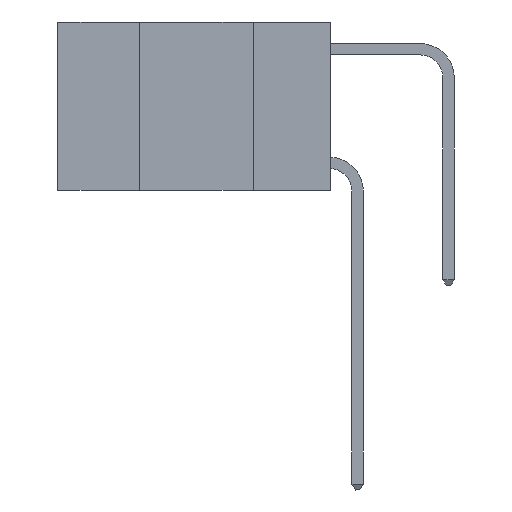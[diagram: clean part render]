
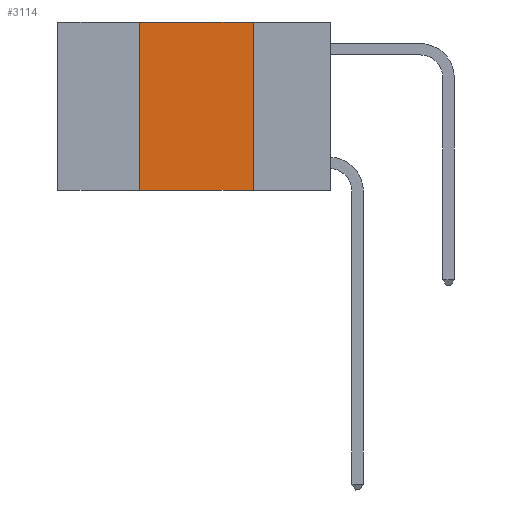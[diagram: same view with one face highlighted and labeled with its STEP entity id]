
A CAD part, left-side view. The second image highlights one B-rep face of the part: STEP entity #3114.
In plain terms, the highlighted planar face has unit normal (-1, 0, 0).
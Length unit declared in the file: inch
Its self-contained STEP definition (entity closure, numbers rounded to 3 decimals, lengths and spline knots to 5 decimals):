
#539 = LINE ( 'NONE', #16491, #15161 ) ;
#803 = VECTOR ( 'NONE', #20908, 39.37008 ) ;
#1067 = EDGE_CURVE ( 'NONE', #13367, #9823, #539, .T. ) ;
#1147 = LINE ( 'NONE', #7611, #14294 ) ;
#1899 = DIRECTION ( 'NONE',  ( 0., 0., -1. ) ) ;
#2015 = DIRECTION ( 'NONE',  ( 0., -1., 0. ) ) ;
#3114 = ADVANCED_FACE ( 'NONE', ( #18063 ), #14567, .F. ) ;
#3498 = DIRECTION ( 'NONE',  ( 0., 0., -1. ) ) ;
#4045 = EDGE_CURVE ( 'NONE', #14087, #9823, #9713, .T. ) ;
#4298 = ORIENTED_EDGE ( 'NONE', *, *, #4045, .T. ) ;
#5186 = AXIS2_PLACEMENT_3D ( 'NONE', #14899, #8161, #3498 ) ;
#7611 = CARTESIAN_POINT ( 'NONE',  ( 0., 0.6, 0. ) ) ;
#7891 = CARTESIAN_POINT ( 'NONE',  ( 0., 0.17, -0.37 ) ) ;
#7904 = CARTESIAN_POINT ( 'NONE',  ( 0., 0.6, -0.37 ) ) ;
#8050 = CARTESIAN_POINT ( 'NONE',  ( 0., 0.42, 0. ) ) ;
#8161 = DIRECTION ( 'NONE',  ( 1., 0., 0. ) ) ;
#9067 = CARTESIAN_POINT ( 'NONE',  ( 0., 0.42, 0. ) ) ;
#9277 = EDGE_CURVE ( 'NONE', #9695, #13367, #1147, .T. ) ;
#9695 = VERTEX_POINT ( 'NONE', #9067 ) ;
#9713 = LINE ( 'NONE', #7904, #803 ) ;
#9823 = VERTEX_POINT ( 'NONE', #7891 ) ;
#10452 = ORIENTED_EDGE ( 'NONE', *, *, #9277, .F. ) ;
#13226 = ORIENTED_EDGE ( 'NONE', *, *, #15278, .F. ) ;
#13367 = VERTEX_POINT ( 'NONE', #19024 ) ;
#13592 = CARTESIAN_POINT ( 'NONE',  ( 0., 0.42, -0.37 ) ) ;
#13761 = ORIENTED_EDGE ( 'NONE', *, *, #1067, .F. ) ;
#14087 = VERTEX_POINT ( 'NONE', #13592 ) ;
#14294 = VECTOR ( 'NONE', #2015, 39.37008 ) ;
#14566 = DIRECTION ( 'NONE',  ( 0., 0., 1. ) ) ;
#14567 = PLANE ( 'NONE',  #5186 ) ;
#14899 = CARTESIAN_POINT ( 'NONE',  ( 0., 0.6, 0. ) ) ;
#15161 = VECTOR ( 'NONE', #1899, 39.37008 ) ;
#15278 = EDGE_CURVE ( 'NONE', #14087, #9695, #20711, .T. ) ;
#16138 = VECTOR ( 'NONE', #14566, 39.37008 ) ;
#16214 = EDGE_LOOP ( 'NONE', ( #13761, #10452, #13226, #4298 ) ) ;
#16491 = CARTESIAN_POINT ( 'NONE',  ( 0., 0.17, 0. ) ) ;
#18063 = FACE_OUTER_BOUND ( 'NONE', #16214, .T. ) ;
#19024 = CARTESIAN_POINT ( 'NONE',  ( 0., 0.17, 0. ) ) ;
#20711 = LINE ( 'NONE', #8050, #16138 ) ;
#20908 = DIRECTION ( 'NONE',  ( 0., -1., 0. ) ) ;
